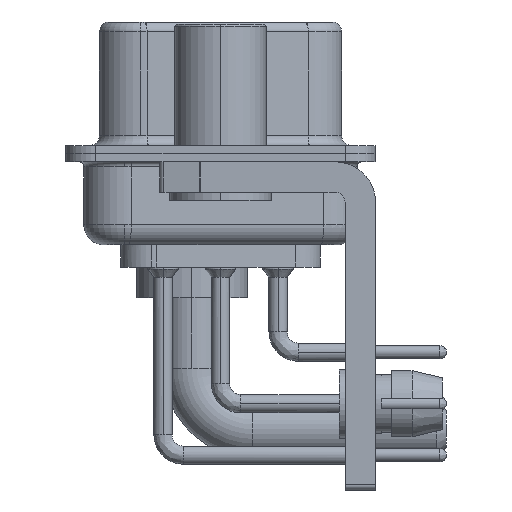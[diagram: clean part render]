
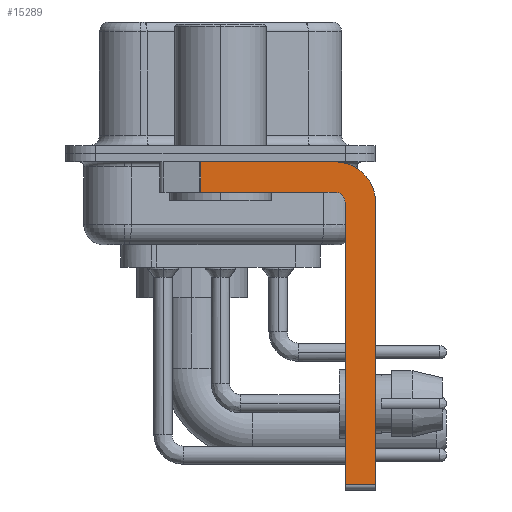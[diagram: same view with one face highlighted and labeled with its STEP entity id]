
A CAD part, left-side view. The second image highlights one B-rep face of the part: STEP entity #15289.
In plain terms, the highlighted planar face has unit normal (-1, 0, 0).
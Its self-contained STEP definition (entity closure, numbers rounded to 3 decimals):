
#121 = CARTESIAN_POINT ( 'NONE',  ( -2.9, -7.65, -16.35 ) ) ;
#458 = AXIS2_PLACEMENT_3D ( 'NONE', #11734, #37351, #32315 ) ;
#639 = ORIENTED_EDGE ( 'NONE', *, *, #16173, .F. ) ;
#2003 = DIRECTION ( 'NONE',  ( 0., 0., -1. ) ) ;
#2093 = VERTEX_POINT ( 'NONE', #12995 ) ;
#2403 = CARTESIAN_POINT ( 'NONE',  ( -2.9, 0.978, -1.9 ) ) ;
#4063 = VERTEX_POINT ( 'NONE', #13613 ) ;
#4893 = CARTESIAN_POINT ( 'NONE',  ( -2.9, -6.15, -16.6 ) ) ;
#4910 = CARTESIAN_POINT ( 'NONE',  ( -2.9, 0.978, -1.9 ) ) ;
#5101 = VERTEX_POINT ( 'NONE', #23386 ) ;
#5573 = VECTOR ( 'NONE', #40388, 1000. ) ;
#5906 = CARTESIAN_POINT ( 'NONE',  ( -2.9, -7.65, -2.4 ) ) ;
#7823 = CIRCLE ( 'NONE', #458, 2. ) ;
#7845 = LINE ( 'NONE', #19834, #15269 ) ;
#7949 = VECTOR ( 'NONE', #31921, 1000. ) ;
#9796 = CARTESIAN_POINT ( 'NONE',  ( -2.9, -5.65, -1.9 ) ) ;
#11385 = ORIENTED_EDGE ( 'NONE', *, *, #32045, .F. ) ;
#11631 = CIRCLE ( 'NONE', #29749, 0.5 ) ;
#11734 = CARTESIAN_POINT ( 'NONE',  ( -2.9, -5.65, -2.4 ) ) ;
#12443 = CARTESIAN_POINT ( 'NONE',  ( -2.9, -7.65, -2.4 ) ) ;
#12995 = CARTESIAN_POINT ( 'NONE',  ( -2.9, -6.15, -2.4 ) ) ;
#13613 = CARTESIAN_POINT ( 'NONE',  ( -2.9, -6.15, -16.35 ) ) ;
#14533 = LINE ( 'NONE', #4893, #5573 ) ;
#15269 = VECTOR ( 'NONE', #23003, 1000. ) ;
#15289 = ADVANCED_FACE ( 'NONE', ( #28278 ), #19007, .F. ) ;
#15392 = EDGE_CURVE ( 'NONE', #32409, #5101, #7845, .T. ) ;
#15768 = ORIENTED_EDGE ( 'NONE', *, *, #25983, .F. ) ;
#15906 = DIRECTION ( 'NONE',  ( 0., 0., 1. ) ) ;
#16173 = EDGE_CURVE ( 'NONE', #5101, #40551, #7823, .T. ) ;
#16294 = VECTOR ( 'NONE', #22756, 1000. ) ;
#16376 = CARTESIAN_POINT ( 'NONE',  ( -2.9, -5.65, -1.9 ) ) ;
#17234 = EDGE_CURVE ( 'NONE', #4063, #18467, #25907, .T. ) ;
#17614 = EDGE_CURVE ( 'NONE', #4063, #2093, #14533, .T. ) ;
#17938 = AXIS2_PLACEMENT_3D ( 'NONE', #19213, #41286, #31839 ) ;
#18467 = VERTEX_POINT ( 'NONE', #121 ) ;
#18495 = ORIENTED_EDGE ( 'NONE', *, *, #21930, .T. ) ;
#19007 = PLANE ( 'NONE',  #17938 ) ;
#19035 = CARTESIAN_POINT ( 'NONE',  ( -2.9, 0.978, -0.4 ) ) ;
#19213 = CARTESIAN_POINT ( 'NONE',  ( -2.9, -5.65, -2.4 ) ) ;
#19834 = CARTESIAN_POINT ( 'NONE',  ( -2.9, 3., -0.4 ) ) ;
#21061 = DIRECTION ( 'NONE',  ( 0., 0., -1. ) ) ;
#21930 = EDGE_CURVE ( 'NONE', #32409, #24457, #30991, .T. ) ;
#22756 = DIRECTION ( 'NONE',  ( 0., -1., 0. ) ) ;
#23003 = DIRECTION ( 'NONE',  ( 0., -1., 0. ) ) ;
#23386 = CARTESIAN_POINT ( 'NONE',  ( -2.9, -5.65, -0.4 ) ) ;
#23390 = VECTOR ( 'NONE', #21061, 1000. ) ;
#23964 = VERTEX_POINT ( 'NONE', #9796 ) ;
#24457 = VERTEX_POINT ( 'NONE', #4910 ) ;
#25907 = LINE ( 'NONE', #31592, #16294 ) ;
#25983 = EDGE_CURVE ( 'NONE', #40551, #18467, #28001, .T. ) ;
#28001 = LINE ( 'NONE', #12443, #23390 ) ;
#28278 = FACE_OUTER_BOUND ( 'NONE', #34122, .T. ) ;
#29391 = LINE ( 'NONE', #16376, #7949 ) ;
#29749 = AXIS2_PLACEMENT_3D ( 'NONE', #35455, #35655, #15906 ) ;
#30991 = LINE ( 'NONE', #2403, #38951 ) ;
#31592 = CARTESIAN_POINT ( 'NONE',  ( -2.9, -5.65, -16.35 ) ) ;
#31839 = DIRECTION ( 'NONE',  ( 0., 0., -1. ) ) ;
#31921 = DIRECTION ( 'NONE',  ( 0., 1., 0. ) ) ;
#32045 = EDGE_CURVE ( 'NONE', #23964, #24457, #29391, .T. ) ;
#32315 = DIRECTION ( 'NONE',  ( 0., 0., -1. ) ) ;
#32409 = VERTEX_POINT ( 'NONE', #19035 ) ;
#32773 = ORIENTED_EDGE ( 'NONE', *, *, #17234, .T. ) ;
#33738 = EDGE_CURVE ( 'NONE', #2093, #23964, #11631, .T. ) ;
#34122 = EDGE_LOOP ( 'NONE', ( #37778, #18495, #11385, #35664, #37572, #32773, #15768, #639 ) ) ;
#35455 = CARTESIAN_POINT ( 'NONE',  ( -2.9, -5.65, -2.4 ) ) ;
#35655 = DIRECTION ( 'NONE',  ( -1., 0., 0. ) ) ;
#35664 = ORIENTED_EDGE ( 'NONE', *, *, #33738, .F. ) ;
#37351 = DIRECTION ( 'NONE',  ( 1., 0., 0. ) ) ;
#37572 = ORIENTED_EDGE ( 'NONE', *, *, #17614, .F. ) ;
#37778 = ORIENTED_EDGE ( 'NONE', *, *, #15392, .F. ) ;
#38951 = VECTOR ( 'NONE', #2003, 1000. ) ;
#40388 = DIRECTION ( 'NONE',  ( 0., 0., 1. ) ) ;
#40551 = VERTEX_POINT ( 'NONE', #5906 ) ;
#41286 = DIRECTION ( 'NONE',  ( 1., 0., 0. ) ) ;
